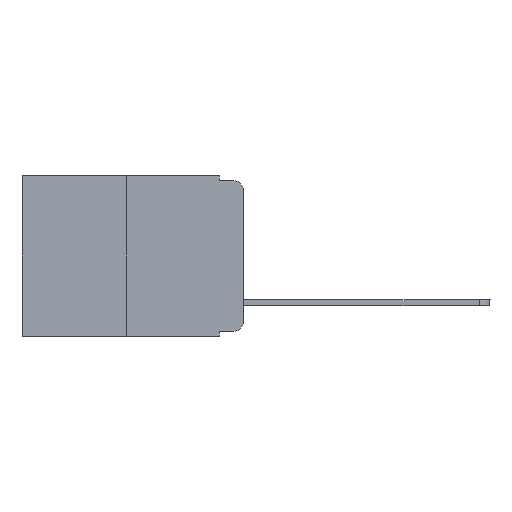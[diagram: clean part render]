
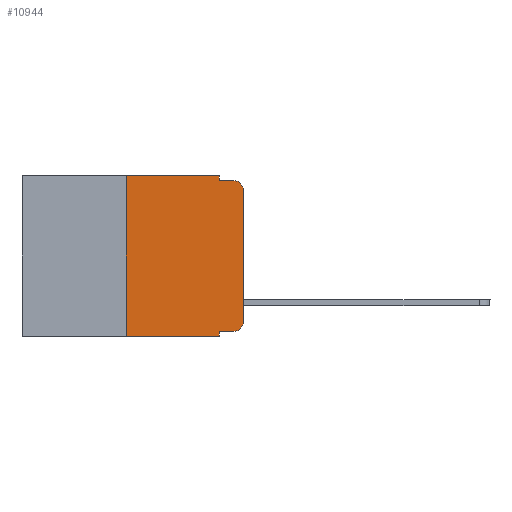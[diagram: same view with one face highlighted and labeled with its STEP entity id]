
A CAD part, left-side view. The second image highlights one B-rep face of the part: STEP entity #10944.
In plain terms, the highlighted planar face has unit normal (-1, 0, 0).
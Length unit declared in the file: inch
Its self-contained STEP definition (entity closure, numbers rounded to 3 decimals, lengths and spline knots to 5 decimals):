
#18 = EDGE_LOOP ( 'NONE', ( #5286, #8197, #4128, #4157, #20020, #20823, #5196, #15626, #21064, #20688 ) ) ;
#148 = CIRCLE ( 'NONE', #7760, 0.02 ) ;
#246 = CARTESIAN_POINT ( 'NONE',  ( 0., 0.02, -0.333 ) ) ;
#270 = VERTEX_POINT ( 'NONE', #22187 ) ;
#525 = AXIS2_PLACEMENT_3D ( 'NONE', #12783, #17909, #7455 ) ;
#1045 = DIRECTION ( 'NONE',  ( 0., -1., 0. ) ) ;
#1254 = CARTESIAN_POINT ( 'NONE',  ( 0., 0.02, -0.01 ) ) ;
#1306 = CARTESIAN_POINT ( 'NONE',  ( 0., 0.051, -0.333 ) ) ;
#2051 = DIRECTION ( 'NONE',  ( -1., 0., 0. ) ) ;
#2633 = DIRECTION ( 'NONE',  ( 0., 0., 1. ) ) ;
#2976 = VECTOR ( 'NONE', #2633, 39.37008 ) ;
#3411 = VECTOR ( 'NONE', #22272, 39.37008 ) ;
#3477 = CIRCLE ( 'NONE', #12246, 0.02 ) ;
#3645 = CARTESIAN_POINT ( 'NONE',  ( 0., 0., -0.03 ) ) ;
#4073 = VERTEX_POINT ( 'NONE', #13170 ) ;
#4128 = ORIENTED_EDGE ( 'NONE', *, *, #18399, .F. ) ;
#4157 = ORIENTED_EDGE ( 'NONE', *, *, #17759, .F. ) ;
#4257 = CARTESIAN_POINT ( 'NONE',  ( 0., 0.473, 0. ) ) ;
#4258 = VERTEX_POINT ( 'NONE', #5492 ) ;
#4266 = VERTEX_POINT ( 'NONE', #9078 ) ;
#4459 = LINE ( 'NONE', #19160, #15782 ) ;
#4560 = VERTEX_POINT ( 'NONE', #21938 ) ;
#4723 = DIRECTION ( 'NONE',  ( 0., 0., -1. ) ) ;
#4885 = DIRECTION ( 'NONE',  ( 0., -1., 0. ) ) ;
#4952 = VECTOR ( 'NONE', #4885, 39.37008 ) ;
#5196 = ORIENTED_EDGE ( 'NONE', *, *, #6019, .T. ) ;
#5286 = ORIENTED_EDGE ( 'NONE', *, *, #21129, .T. ) ;
#5492 = CARTESIAN_POINT ( 'NONE',  ( 0., 0., -0.313 ) ) ;
#5556 = CARTESIAN_POINT ( 'NONE',  ( 0., 0.02, -0.03 ) ) ;
#5646 = DIRECTION ( 'NONE',  ( 0., 0., -1. ) ) ;
#5690 = CARTESIAN_POINT ( 'NONE',  ( 0., 0.473, -0.343 ) ) ;
#6019 = EDGE_CURVE ( 'NONE', #13491, #270, #14790, .T. ) ;
#7455 = DIRECTION ( 'NONE',  ( 0., 0., -1. ) ) ;
#7760 = AXIS2_PLACEMENT_3D ( 'NONE', #9908, #11687, #19265 ) ;
#8101 = LINE ( 'NONE', #22044, #3411 ) ;
#8197 = ORIENTED_EDGE ( 'NONE', *, *, #16075, .T. ) ;
#9078 = CARTESIAN_POINT ( 'NONE',  ( 0., 0.051, -0.01 ) ) ;
#9177 = EDGE_CURVE ( 'NONE', #4073, #22155, #18442, .T. ) ;
#9296 = CARTESIAN_POINT ( 'NONE',  ( 0., 0.25, -0.343 ) ) ;
#9337 = EDGE_CURVE ( 'NONE', #4073, #270, #11866, .T. ) ;
#9338 = DIRECTION ( 'NONE',  ( 0., -1., 0. ) ) ;
#9908 = CARTESIAN_POINT ( 'NONE',  ( 0., 0.02, -0.313 ) ) ;
#9983 = CARTESIAN_POINT ( 'NONE',  ( 0., 0.051, 0. ) ) ;
#10944 = ADVANCED_FACE ( 'NONE', ( #17234 ), #17996, .F. ) ;
#11687 = DIRECTION ( 'NONE',  ( -1., 0., 0. ) ) ;
#11866 = LINE ( 'NONE', #15924, #20651 ) ;
#11985 = EDGE_CURVE ( 'NONE', #22155, #4258, #148, .T. ) ;
#12226 = VECTOR ( 'NONE', #4723, 39.37008 ) ;
#12246 = AXIS2_PLACEMENT_3D ( 'NONE', #5556, #2051, #21339 ) ;
#12562 = VECTOR ( 'NONE', #9338, 39.37008 ) ;
#12783 = CARTESIAN_POINT ( 'NONE',  ( 0., 0.473, 0. ) ) ;
#12876 = LINE ( 'NONE', #4257, #16740 ) ;
#13170 = CARTESIAN_POINT ( 'NONE',  ( 0., 0.051, -0.333 ) ) ;
#13491 = VERTEX_POINT ( 'NONE', #9296 ) ;
#14790 = LINE ( 'NONE', #5690, #12562 ) ;
#15108 = VERTEX_POINT ( 'NONE', #3645 ) ;
#15498 = EDGE_CURVE ( 'NONE', #20544, #4560, #12876, .T. ) ;
#15626 = ORIENTED_EDGE ( 'NONE', *, *, #9337, .F. ) ;
#15782 = VECTOR ( 'NONE', #22476, 39.37008 ) ;
#15924 = CARTESIAN_POINT ( 'NONE',  ( 0., 0.051, 0. ) ) ;
#16075 = EDGE_CURVE ( 'NONE', #15108, #19562, #3477, .T. ) ;
#16740 = VECTOR ( 'NONE', #1045, 39.37008 ) ;
#16904 = LINE ( 'NONE', #9983, #12226 ) ;
#17234 = FACE_OUTER_BOUND ( 'NONE', #18, .T. ) ;
#17719 = EDGE_CURVE ( 'NONE', #13491, #20544, #8101, .T. ) ;
#17759 = EDGE_CURVE ( 'NONE', #4560, #4266, #16904, .T. ) ;
#17909 = DIRECTION ( 'NONE',  ( 1., 0., 0. ) ) ;
#17996 = PLANE ( 'NONE',  #525 ) ;
#18313 = CARTESIAN_POINT ( 'NONE',  ( 0., 0., 0. ) ) ;
#18399 = EDGE_CURVE ( 'NONE', #4266, #19562, #4459, .T. ) ;
#18442 = LINE ( 'NONE', #1306, #4952 ) ;
#18669 = LINE ( 'NONE', #18313, #2976 ) ;
#19160 = CARTESIAN_POINT ( 'NONE',  ( 0., 0.051, -0.01 ) ) ;
#19265 = DIRECTION ( 'NONE',  ( 0., 0., -1. ) ) ;
#19562 = VERTEX_POINT ( 'NONE', #1254 ) ;
#20020 = ORIENTED_EDGE ( 'NONE', *, *, #15498, .F. ) ;
#20544 = VERTEX_POINT ( 'NONE', #22125 ) ;
#20651 = VECTOR ( 'NONE', #5646, 39.37008 ) ;
#20688 = ORIENTED_EDGE ( 'NONE', *, *, #11985, .T. ) ;
#20823 = ORIENTED_EDGE ( 'NONE', *, *, #17719, .F. ) ;
#21064 = ORIENTED_EDGE ( 'NONE', *, *, #9177, .T. ) ;
#21129 = EDGE_CURVE ( 'NONE', #4258, #15108, #18669, .T. ) ;
#21339 = DIRECTION ( 'NONE',  ( 0., 0., -1. ) ) ;
#21938 = CARTESIAN_POINT ( 'NONE',  ( 0., 0.051, 0. ) ) ;
#22044 = CARTESIAN_POINT ( 'NONE',  ( 0., 0.25, 0. ) ) ;
#22125 = CARTESIAN_POINT ( 'NONE',  ( 0., 0.25, 0. ) ) ;
#22155 = VERTEX_POINT ( 'NONE', #246 ) ;
#22187 = CARTESIAN_POINT ( 'NONE',  ( 0., 0.051, -0.343 ) ) ;
#22272 = DIRECTION ( 'NONE',  ( 0., 0., 1. ) ) ;
#22476 = DIRECTION ( 'NONE',  ( 0., -1., 0. ) ) ;
